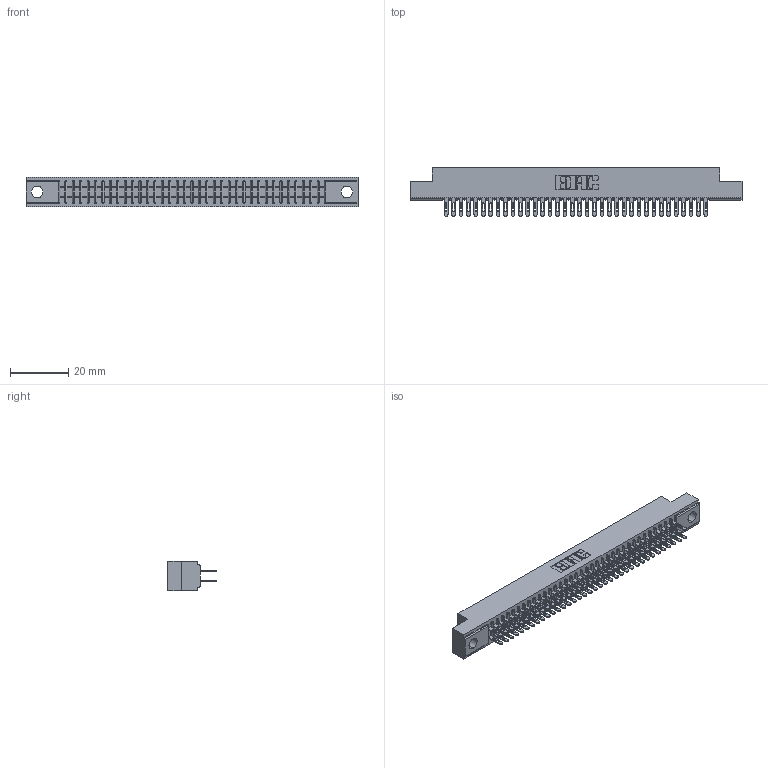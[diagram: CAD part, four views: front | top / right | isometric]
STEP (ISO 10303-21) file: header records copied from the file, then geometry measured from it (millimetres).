
FILE_DESCRIPTION (( 'STEP AP203' ), '1' );
FILE_NAME ('341-072-500-204.STEP', '2018-08-07T19:47:01', ( '' ), ( '' ), 'SwSTEP 2.0', 'SolidWorks 2016', '' );
FILE_SCHEMA (( 'CONFIG_CONTROL_DESIGN' ));
Length unit declared in the file: inch
Products named in the file (3): 341 Part_.156 (3.96) Dia Mounting Holes; 341-292-001_341-292-100; 341-072-500-204
Assembly tree (73 placements, depth 2):
  341-072-500-204
    341 Part_.156 (3.96) Dia Mounting Holes
    341-292-001_341-292-100  x72
Bounding box: 113.67 x 16.69 x 10.16 mm (x, y, z)
Volume: 8375.3 mm3; surface area: 15164.6 mm2
Topology: 73 solids, 73 shells, 4882 faces, 14140 edges, 9158 vertices
Faces by surface type: plane 2818, cylinder 1920, sphere 74, torus 70
Entity records: 44793 total; most frequent: CARTESIAN_POINT 7450, ORIENTED_EDGE 7400, DIRECTION 7230, EDGE_CURVE 3700, LINE 2986, VECTOR 2986, VERTEX_POINT 2342, AXIS2_PLACEMENT_3D 2122
